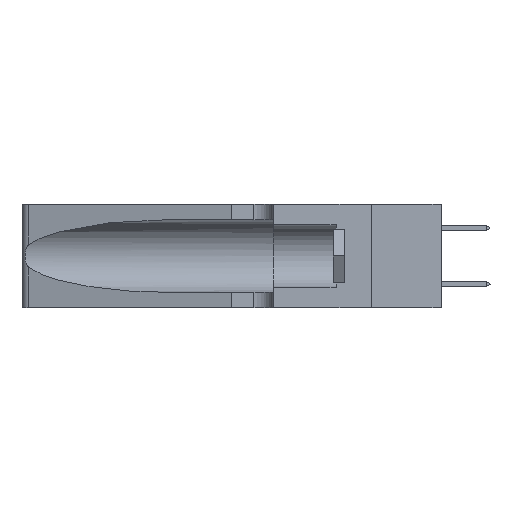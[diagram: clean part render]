
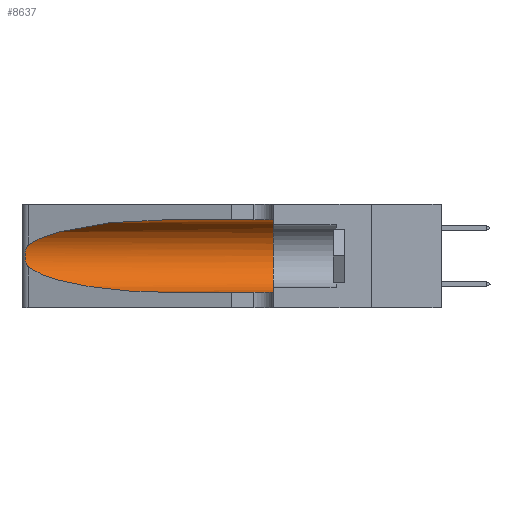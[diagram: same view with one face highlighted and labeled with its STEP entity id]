
A CAD part, left-side view. The second image highlights one B-rep face of the part: STEP entity #8637.
In plain terms, the highlighted cylindrical face has radius 3.308 mm (diameter 6.617 mm), a partial arc.
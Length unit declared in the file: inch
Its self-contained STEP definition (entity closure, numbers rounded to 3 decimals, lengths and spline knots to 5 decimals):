
#379 = CARTESIAN_POINT ( 'NONE',  ( 0.1305, 0.72297, 0.31525 ) ) ;
#480 = LINE ( 'NONE', #12264, #17355 ) ;
#528 = LINE ( 'NONE', #8064, #6520 ) ;
#1012 = CARTESIAN_POINT ( 'NONE',  ( 0.26075, 1.23896, 0.19203 ) ) ;
#1053 = CARTESIAN_POINT ( 'NONE',  ( 0.25487, 1.22718, 0.14631 ) ) ;
#1315 = CARTESIAN_POINT ( 'NONE',  ( 0.25856, 1.23593, 0.16098 ) ) ;
#1384 =( BOUNDED_CURVE ( )  B_SPLINE_CURVE ( 3, ( #1053, #17665, #14868, #12132 ),
 .UNSPECIFIED., .F., .F. ) 
 B_SPLINE_CURVE_WITH_KNOTS ( ( 4, 4 ),
 ( 3.44316, 4.71239 ),
 .UNSPECIFIED. ) 
 CURVE ( )  GEOMETRIC_REPRESENTATION_ITEM ( )  RATIONAL_B_SPLINE_CURVE ( ( 1., 0.87, 0.87, 1. ) ) 
 REPRESENTATION_ITEM ( '' )  );
#1481 = VERTEX_POINT ( 'NONE', #15996 ) ;
#1491 = FACE_OUTER_BOUND ( 'NONE', #11678, .T. ) ;
#2063 = CIRCLE ( 'NONE', #6821, 0.13025 ) ;
#2701 = CARTESIAN_POINT ( 'NONE',  ( 0.25854, 1.2359, 0.20912 ) ) ;
#3656 = CARTESIAN_POINT ( 'NONE',  ( 0.25787, 1.23484, 0.2124 ) ) ;
#4096 = CARTESIAN_POINT ( 'NONE',  ( 0.25639, 1.23186, 0.15144 ) ) ;
#4105 = EDGE_CURVE ( 'NONE', #9514, #1481, #1384, .T. ) ;
#4292 = CARTESIAN_POINT ( 'NONE',  ( 0.1305, 0.35, 0.05475 ) ) ;
#4843 = AXIS2_PLACEMENT_3D ( 'NONE', #13586, #5406, #16423 ) ;
#5070 = ORIENTED_EDGE ( 'NONE', *, *, #6992, .T. ) ;
#5406 = DIRECTION ( 'NONE',  ( 0., -1., 0. ) ) ;
#5524 = CARTESIAN_POINT ( 'NONE',  ( 0.25487, 1.22718, 0.22369 ) ) ;
#5868 = ORIENTED_EDGE ( 'NONE', *, *, #9884, .F. ) ;
#5915 = B_SPLINE_CURVE_WITH_KNOTS ( 'NONE', 3,
 ( #11979, #9160, #12280, #3656, #2701, #9534, #1012, #14583, #10600, #1315, #6409, #4096, #13636, #15943 ),
 .UNSPECIFIED., .F., .F.,
 ( 4, 2, 2, 2, 2, 2, 4 ),
 ( 0., 0.00027, 0.00053, 0.00107, 0.0016, 0.00187, 0.00214 ),
 .UNSPECIFIED. ) ;
#6290 = ORIENTED_EDGE ( 'NONE', *, *, #6793, .T. ) ;
#6323 = VERTEX_POINT ( 'NONE', #5524 ) ;
#6409 = CARTESIAN_POINT ( 'NONE',  ( 0.25789, 1.23486, 0.15765 ) ) ;
#6520 = VECTOR ( 'NONE', #13502, 39.37008 ) ;
#6793 = EDGE_CURVE ( 'NONE', #16288, #6323, #14418, .T. ) ;
#6821 = AXIS2_PLACEMENT_3D ( 'NONE', #7373, #12754, #14108 ) ;
#6992 = EDGE_CURVE ( 'NONE', #1481, #8143, #528, .T. ) ;
#7373 = CARTESIAN_POINT ( 'NONE',  ( 0.1305, 0.35, 0.185 ) ) ;
#7578 = EDGE_CURVE ( 'NONE', #6323, #9514, #5915, .T. ) ;
#7697 = CYLINDRICAL_SURFACE ( 'NONE', #4843, 0.13025 ) ;
#8064 = CARTESIAN_POINT ( 'NONE',  ( 0.1305, 1.61858, 0.05475 ) ) ;
#8128 = VERTEX_POINT ( 'NONE', #13834 ) ;
#8143 = VERTEX_POINT ( 'NONE', #4292 ) ;
#8378 = ORIENTED_EDGE ( 'NONE', *, *, #13260, .F. ) ;
#8599 = CARTESIAN_POINT ( 'NONE',  ( 0.1305, 0.72297, 0.31525 ) ) ;
#8637 = ADVANCED_FACE ( 'NONE', ( #1491 ), #7697, .F. ) ;
#8737 = ORIENTED_EDGE ( 'NONE', *, *, #4105, .T. ) ;
#9160 = CARTESIAN_POINT ( 'NONE',  ( 0.25555, 1.22994, 0.2215 ) ) ;
#9514 = VERTEX_POINT ( 'NONE', #11773 ) ;
#9534 = CARTESIAN_POINT ( 'NONE',  ( 0.26018, 1.23835, 0.19895 ) ) ;
#9884 = EDGE_CURVE ( 'NONE', #8128, #8143, #2063, .T. ) ;
#10080 = CARTESIAN_POINT ( 'NONE',  ( 0.18966, 0.96281, 0.31525 ) ) ;
#10600 = CARTESIAN_POINT ( 'NONE',  ( 0.26017, 1.23833, 0.17102 ) ) ;
#10731 = ORIENTED_EDGE ( 'NONE', *, *, #7578, .T. ) ;
#11678 = EDGE_LOOP ( 'NONE', ( #6290, #10731, #8737, #5070, #5868, #8378 ) ) ;
#11773 = CARTESIAN_POINT ( 'NONE',  ( 0.25487, 1.22718, 0.14631 ) ) ;
#11979 = CARTESIAN_POINT ( 'NONE',  ( 0.25487, 1.22718, 0.22369 ) ) ;
#12132 = CARTESIAN_POINT ( 'NONE',  ( 0.1305, 0.72297, 0.05475 ) ) ;
#12264 = CARTESIAN_POINT ( 'NONE',  ( 0.1305, 1.61858, 0.31525 ) ) ;
#12280 = CARTESIAN_POINT ( 'NONE',  ( 0.25639, 1.23184, 0.21858 ) ) ;
#12754 = DIRECTION ( 'NONE',  ( 0., 1., 0. ) ) ;
#13260 = EDGE_CURVE ( 'NONE', #16288, #8128, #480, .T. ) ;
#13472 = CARTESIAN_POINT ( 'NONE',  ( 0.2373, 1.15595, 0.28018 ) ) ;
#13502 = DIRECTION ( 'NONE',  ( 0., -1., 0. ) ) ;
#13586 = CARTESIAN_POINT ( 'NONE',  ( 0.1305, 1.61858, 0.185 ) ) ;
#13636 = CARTESIAN_POINT ( 'NONE',  ( 0.25555, 1.22993, 0.14849 ) ) ;
#13739 = DIRECTION ( 'NONE',  ( 0., -1., 0. ) ) ;
#13834 = CARTESIAN_POINT ( 'NONE',  ( 0.1305, 0.35, 0.31525 ) ) ;
#14108 = DIRECTION ( 'NONE',  ( 0., 0., 1. ) ) ;
#14418 =( BOUNDED_CURVE ( )  B_SPLINE_CURVE ( 3, ( #379, #10080, #13472, #14839 ),
 .UNSPECIFIED., .F., .F. ) 
 B_SPLINE_CURVE_WITH_KNOTS ( ( 4, 4 ),
 ( 1.5708, 2.84003 ),
 .UNSPECIFIED. ) 
 CURVE ( )  GEOMETRIC_REPRESENTATION_ITEM ( )  RATIONAL_B_SPLINE_CURVE ( ( 1., 0.87, 0.87, 1. ) ) 
 REPRESENTATION_ITEM ( '' )  );
#14583 = CARTESIAN_POINT ( 'NONE',  ( 0.26075, 1.23896, 0.178 ) ) ;
#14839 = CARTESIAN_POINT ( 'NONE',  ( 0.25487, 1.22718, 0.22369 ) ) ;
#14868 = CARTESIAN_POINT ( 'NONE',  ( 0.18966, 0.96281, 0.05475 ) ) ;
#15943 = CARTESIAN_POINT ( 'NONE',  ( 0.25487, 1.22718, 0.14631 ) ) ;
#15996 = CARTESIAN_POINT ( 'NONE',  ( 0.1305, 0.72297, 0.05475 ) ) ;
#16288 = VERTEX_POINT ( 'NONE', #8599 ) ;
#16423 = DIRECTION ( 'NONE',  ( 0., 0., -1. ) ) ;
#17355 = VECTOR ( 'NONE', #13739, 39.37008 ) ;
#17665 = CARTESIAN_POINT ( 'NONE',  ( 0.2373, 1.15595, 0.08982 ) ) ;
